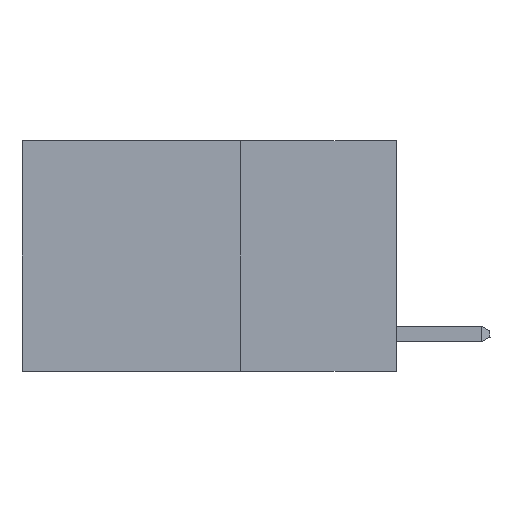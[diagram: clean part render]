
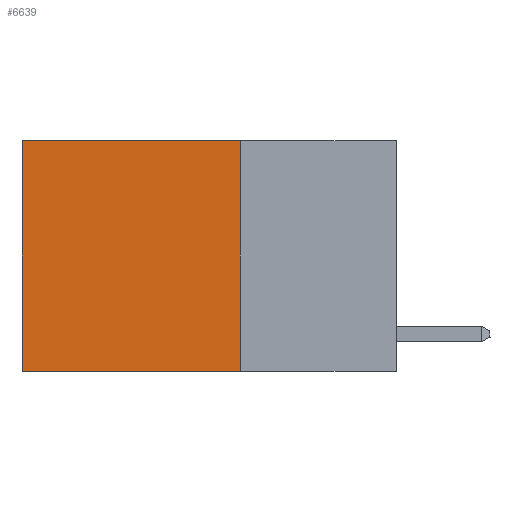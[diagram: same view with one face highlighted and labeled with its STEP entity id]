
A CAD part, left-side view. The second image highlights one B-rep face of the part: STEP entity #6639.
In plain terms, the highlighted planar face has unit normal (-1, 0, 0).
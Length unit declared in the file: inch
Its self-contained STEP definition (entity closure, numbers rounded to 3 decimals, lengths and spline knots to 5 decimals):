
#247 = LINE ( 'NONE', #7688, #2738 ) ;
#262 = EDGE_LOOP ( 'NONE', ( #4750, #4208, #1853, #2730 ) ) ;
#366 = CARTESIAN_POINT ( 'NONE',  ( 0.2625, 0.25, 0. ) ) ;
#402 = CARTESIAN_POINT ( 'NONE',  ( 0.2625, 0.25, 0. ) ) ;
#1456 = LINE ( 'NONE', #2176, #1970 ) ;
#1567 = CARTESIAN_POINT ( 'NONE',  ( 0.2625, 0.25, 0. ) ) ;
#1702 = VECTOR ( 'NONE', #9202, 39.37008 ) ;
#1853 = ORIENTED_EDGE ( 'NONE', *, *, #7428, .F. ) ;
#1970 = VECTOR ( 'NONE', #8842, 39.37008 ) ;
#2176 = CARTESIAN_POINT ( 'NONE',  ( 0.2625, 0.25, 0. ) ) ;
#2730 = ORIENTED_EDGE ( 'NONE', *, *, #6977, .T. ) ;
#2738 = VECTOR ( 'NONE', #9518, 39.37008 ) ;
#3332 = VERTEX_POINT ( 'NONE', #1567 ) ;
#3745 = CARTESIAN_POINT ( 'NONE',  ( 0.2625, 0.25, -0.37 ) ) ;
#3969 = PLANE ( 'NONE',  #10051 ) ;
#4208 = ORIENTED_EDGE ( 'NONE', *, *, #6091, .F. ) ;
#4750 = ORIENTED_EDGE ( 'NONE', *, *, #6884, .T. ) ;
#4852 = VERTEX_POINT ( 'NONE', #11238 ) ;
#5015 = CARTESIAN_POINT ( 'NONE',  ( 0.2625, 0.25, -0.37 ) ) ;
#5042 = VECTOR ( 'NONE', #5046, 39.37008 ) ;
#5046 = DIRECTION ( 'NONE',  ( 0., 0., -1. ) ) ;
#6091 = EDGE_CURVE ( 'NONE', #8271, #8338, #8345, .T. ) ;
#6288 = CARTESIAN_POINT ( 'NONE',  ( 0.2625, 0.6, -0.37 ) ) ;
#6639 = ADVANCED_FACE ( 'NONE', ( #8682 ), #3969, .F. ) ;
#6843 = DIRECTION ( 'NONE',  ( 0., 0., -1. ) ) ;
#6884 = EDGE_CURVE ( 'NONE', #4852, #8338, #247, .T. ) ;
#6977 = EDGE_CURVE ( 'NONE', #3332, #4852, #1456, .T. ) ;
#7428 = EDGE_CURVE ( 'NONE', #3332, #8271, #9631, .T. ) ;
#7688 = CARTESIAN_POINT ( 'NONE',  ( 0.2625, 0.6, 0. ) ) ;
#7768 = DIRECTION ( 'NONE',  ( 1., 0., 0. ) ) ;
#8271 = VERTEX_POINT ( 'NONE', #5015 ) ;
#8338 = VERTEX_POINT ( 'NONE', #6288 ) ;
#8345 = LINE ( 'NONE', #3745, #1702 ) ;
#8682 = FACE_OUTER_BOUND ( 'NONE', #262, .T. ) ;
#8842 = DIRECTION ( 'NONE',  ( 0., 1., 0. ) ) ;
#9202 = DIRECTION ( 'NONE',  ( 0., 1., 0. ) ) ;
#9518 = DIRECTION ( 'NONE',  ( 0., 0., -1. ) ) ;
#9631 = LINE ( 'NONE', #366, #5042 ) ;
#10051 = AXIS2_PLACEMENT_3D ( 'NONE', #402, #7768, #6843 ) ;
#11238 = CARTESIAN_POINT ( 'NONE',  ( 0.2625, 0.6, 0. ) ) ;
